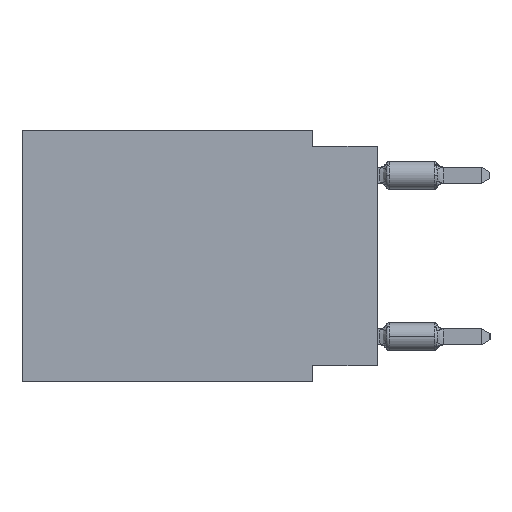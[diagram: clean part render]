
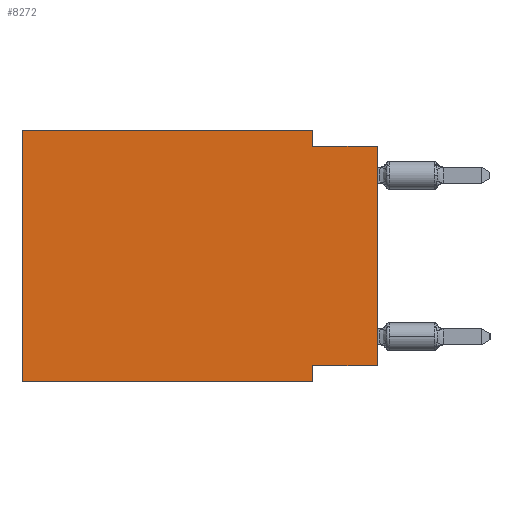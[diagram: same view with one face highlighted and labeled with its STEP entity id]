
A CAD part, left-side view. The second image highlights one B-rep face of the part: STEP entity #8272.
In plain terms, the highlighted planar face has unit normal (-1, 0, 0).
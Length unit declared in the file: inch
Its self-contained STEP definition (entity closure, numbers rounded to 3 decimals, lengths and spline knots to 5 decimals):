
#120 = LINE ( 'NONE', #46564, #5601 ) ;
#768 = EDGE_LOOP ( 'NONE', ( #42950, #39637, #2484, #27123, #33105, #22586, #28189, #11826 ) ) ;
#918 = VERTEX_POINT ( 'NONE', #2044 ) ;
#1153 = EDGE_CURVE ( 'NONE', #2080, #918, #120, .T. ) ;
#2044 = CARTESIAN_POINT ( 'NONE',  ( 0., 0.1, -0.39 ) ) ;
#2080 = VERTEX_POINT ( 'NONE', #4877 ) ;
#2137 = VECTOR ( 'NONE', #12188, 39.37008 ) ;
#2150 = EDGE_CURVE ( 'NONE', #32019, #34190, #26988, .T. ) ;
#2484 = ORIENTED_EDGE ( 'NONE', *, *, #8875, .F. ) ;
#3300 = DIRECTION ( 'NONE',  ( 0., 1., 0. ) ) ;
#4662 = LINE ( 'NONE', #40253, #46068 ) ;
#4877 = CARTESIAN_POINT ( 'NONE',  ( 0., 0.55, -0.39 ) ) ;
#5081 = DIRECTION ( 'NONE',  ( 0., 0., 1. ) ) ;
#5182 = CARTESIAN_POINT ( 'NONE',  ( 0., 0.55, 0. ) ) ;
#5601 = VECTOR ( 'NONE', #36151, 39.37008 ) ;
#6518 = VERTEX_POINT ( 'NONE', #39132 ) ;
#7536 = CARTESIAN_POINT ( 'NONE',  ( 0., 0., -0.365 ) ) ;
#8272 = ADVANCED_FACE ( 'NONE', ( #13784 ), #28156, .F. ) ;
#8875 = EDGE_CURVE ( 'NONE', #6518, #32019, #27570, .T. ) ;
#11364 = CARTESIAN_POINT ( 'NONE',  ( 0., 0.55, 0. ) ) ;
#11826 = ORIENTED_EDGE ( 'NONE', *, *, #16581, .F. ) ;
#11956 = DIRECTION ( 'NONE',  ( 0., -1., 0. ) ) ;
#12188 = DIRECTION ( 'NONE',  ( 0., 0., -1. ) ) ;
#13784 = FACE_OUTER_BOUND ( 'NONE', #768, .T. ) ;
#14577 = VECTOR ( 'NONE', #3300, 39.37008 ) ;
#14812 = LINE ( 'NONE', #7536, #14577 ) ;
#15490 = VERTEX_POINT ( 'NONE', #36738 ) ;
#15570 = VECTOR ( 'NONE', #16446, 39.37008 ) ;
#15919 = CARTESIAN_POINT ( 'NONE',  ( 0., 0.1, -0.39 ) ) ;
#16111 = CARTESIAN_POINT ( 'NONE',  ( 0., 0., 0. ) ) ;
#16446 = DIRECTION ( 'NONE',  ( 0., -1., 0. ) ) ;
#16579 = LINE ( 'NONE', #16111, #21690 ) ;
#16581 = EDGE_CURVE ( 'NONE', #42227, #15490, #14812, .T. ) ;
#18476 = AXIS2_PLACEMENT_3D ( 'NONE', #42557, #35454, #28381 ) ;
#19002 = DIRECTION ( 'NONE',  ( 0., 0., 1. ) ) ;
#19223 = LINE ( 'NONE', #15919, #2137 ) ;
#21629 = EDGE_CURVE ( 'NONE', #15490, #918, #19223, .T. ) ;
#21690 = VECTOR ( 'NONE', #5081, 39.37008 ) ;
#22586 = ORIENTED_EDGE ( 'NONE', *, *, #1153, .T. ) ;
#23309 = EDGE_CURVE ( 'NONE', #42227, #34190, #16579, .T. ) ;
#25222 = VERTEX_POINT ( 'NONE', #11364 ) ;
#26726 = CARTESIAN_POINT ( 'NONE',  ( 0., 0., -0.025 ) ) ;
#26988 = LINE ( 'NONE', #44713, #33497 ) ;
#27123 = ORIENTED_EDGE ( 'NONE', *, *, #32223, .F. ) ;
#27570 = LINE ( 'NONE', #45065, #33994 ) ;
#27599 = EDGE_CURVE ( 'NONE', #2080, #25222, #4662, .T. ) ;
#28156 = PLANE ( 'NONE',  #18476 ) ;
#28189 = ORIENTED_EDGE ( 'NONE', *, *, #21629, .F. ) ;
#28381 = DIRECTION ( 'NONE',  ( 0., 0., -1. ) ) ;
#32019 = VERTEX_POINT ( 'NONE', #35581 ) ;
#32223 = EDGE_CURVE ( 'NONE', #25222, #6518, #33895, .T. ) ;
#33105 = ORIENTED_EDGE ( 'NONE', *, *, #27599, .F. ) ;
#33497 = VECTOR ( 'NONE', #11956, 39.37008 ) ;
#33895 = LINE ( 'NONE', #5182, #15570 ) ;
#33994 = VECTOR ( 'NONE', #45295, 39.37008 ) ;
#34190 = VERTEX_POINT ( 'NONE', #26726 ) ;
#35454 = DIRECTION ( 'NONE',  ( 1., 0., 0. ) ) ;
#35581 = CARTESIAN_POINT ( 'NONE',  ( 0., 0.1, -0.025 ) ) ;
#36151 = DIRECTION ( 'NONE',  ( 0., -1., 0. ) ) ;
#36738 = CARTESIAN_POINT ( 'NONE',  ( 0., 0.1, -0.365 ) ) ;
#37351 = CARTESIAN_POINT ( 'NONE',  ( 0., 0., -0.365 ) ) ;
#39132 = CARTESIAN_POINT ( 'NONE',  ( 0., 0.1, 0. ) ) ;
#39637 = ORIENTED_EDGE ( 'NONE', *, *, #2150, .F. ) ;
#40253 = CARTESIAN_POINT ( 'NONE',  ( 0., 0.55, 0. ) ) ;
#42227 = VERTEX_POINT ( 'NONE', #37351 ) ;
#42557 = CARTESIAN_POINT ( 'NONE',  ( 0., 0.55, 0. ) ) ;
#42950 = ORIENTED_EDGE ( 'NONE', *, *, #23309, .T. ) ;
#44713 = CARTESIAN_POINT ( 'NONE',  ( 0., 0., -0.025 ) ) ;
#45065 = CARTESIAN_POINT ( 'NONE',  ( 0., 0.1, 0. ) ) ;
#45295 = DIRECTION ( 'NONE',  ( 0., 0., -1. ) ) ;
#46068 = VECTOR ( 'NONE', #19002, 39.37008 ) ;
#46564 = CARTESIAN_POINT ( 'NONE',  ( 0., 0.55, -0.39 ) ) ;
